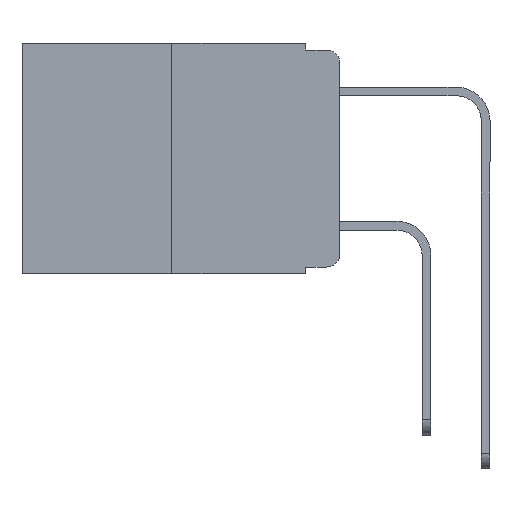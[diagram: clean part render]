
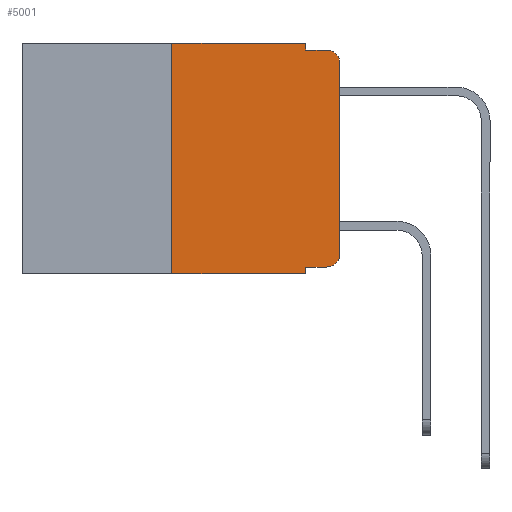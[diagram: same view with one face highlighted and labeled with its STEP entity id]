
A CAD part, left-side view. The second image highlights one B-rep face of the part: STEP entity #5001.
In plain terms, the highlighted planar face has unit normal (-1, 0, 0).
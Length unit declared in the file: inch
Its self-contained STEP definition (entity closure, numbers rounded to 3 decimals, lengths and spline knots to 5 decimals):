
#35 = ORIENTED_EDGE ( 'NONE', *, *, #887, .T. ) ;
#97 = VECTOR ( 'NONE', #2589, 39.37008 ) ;
#420 = DIRECTION ( 'NONE',  ( 0., 0., -1. ) ) ;
#448 = DIRECTION ( 'NONE',  ( 1., 0., 0. ) ) ;
#576 = VECTOR ( 'NONE', #7591, 39.37008 ) ;
#628 = CARTESIAN_POINT ( 'NONE',  ( 0., 0.051, 0. ) ) ;
#778 = LINE ( 'NONE', #7383, #7174 ) ;
#887 = EDGE_CURVE ( 'NONE', #8744, #9918, #8499, .T. ) ;
#1241 = CARTESIAN_POINT ( 'NONE',  ( 0., 0.051, -0.333 ) ) ;
#1350 = LINE ( 'NONE', #6227, #8189 ) ;
#1382 = CARTESIAN_POINT ( 'NONE',  ( 0., 0.02, -0.333 ) ) ;
#1446 = CARTESIAN_POINT ( 'NONE',  ( 0., 0., -0.313 ) ) ;
#1821 = DIRECTION ( 'NONE',  ( 0., -1., 0. ) ) ;
#2236 = PLANE ( 'NONE',  #8236 ) ;
#2323 = VERTEX_POINT ( 'NONE', #5712 ) ;
#2476 = CARTESIAN_POINT ( 'NONE',  ( 0., 0.25, -0.343 ) ) ;
#2589 = DIRECTION ( 'NONE',  ( 0., 0., -1. ) ) ;
#2742 = EDGE_CURVE ( 'NONE', #6399, #9145, #3777, .T. ) ;
#2753 = VERTEX_POINT ( 'NONE', #3191 ) ;
#2765 = CARTESIAN_POINT ( 'NONE',  ( 0., 0.02, -0.03 ) ) ;
#3017 = LINE ( 'NONE', #628, #576 ) ;
#3191 = CARTESIAN_POINT ( 'NONE',  ( 0., 0.25, 0. ) ) ;
#3298 = LINE ( 'NONE', #5934, #7515 ) ;
#3636 = DIRECTION ( 'NONE',  ( 0., 0., -1. ) ) ;
#3777 = LINE ( 'NONE', #4239, #6060 ) ;
#4095 = AXIS2_PLACEMENT_3D ( 'NONE', #2765, #8612, #3636 ) ;
#4237 = DIRECTION ( 'NONE',  ( -1., 0., 0. ) ) ;
#4239 = CARTESIAN_POINT ( 'NONE',  ( 0., 0.473, -0.343 ) ) ;
#4257 = FACE_OUTER_BOUND ( 'NONE', #5559, .T. ) ;
#4327 = VERTEX_POINT ( 'NONE', #1446 ) ;
#4471 = ORIENTED_EDGE ( 'NONE', *, *, #4555, .F. ) ;
#4555 = EDGE_CURVE ( 'NONE', #2323, #5750, #1350, .T. ) ;
#4623 = CARTESIAN_POINT ( 'NONE',  ( 0., 0.051, 0. ) ) ;
#4671 = EDGE_CURVE ( 'NONE', #2753, #8666, #778, .T. ) ;
#4885 = ORIENTED_EDGE ( 'NONE', *, *, #4671, .F. ) ;
#5001 = ADVANCED_FACE ( 'NONE', ( #4257 ), #2236, .F. ) ;
#5395 = ORIENTED_EDGE ( 'NONE', *, *, #9504, .F. ) ;
#5559 = EDGE_LOOP ( 'NONE', ( #5754, #6509, #4471, #5395, #4885, #10902, #8084, #10586, #35, #9125 ) ) ;
#5712 = CARTESIAN_POINT ( 'NONE',  ( 0., 0.051, -0.01 ) ) ;
#5750 = VERTEX_POINT ( 'NONE', #9078 ) ;
#5754 = ORIENTED_EDGE ( 'NONE', *, *, #9727, .T. ) ;
#5934 = CARTESIAN_POINT ( 'NONE',  ( 0., 0.25, 0. ) ) ;
#6060 = VECTOR ( 'NONE', #6420, 39.37008 ) ;
#6080 = DIRECTION ( 'NONE',  ( 0., -1., 0. ) ) ;
#6099 = CARTESIAN_POINT ( 'NONE',  ( 0., 0.473, 0. ) ) ;
#6188 = AXIS2_PLACEMENT_3D ( 'NONE', #9131, #4237, #9923 ) ;
#6193 = DIRECTION ( 'NONE',  ( 0., -1., 0. ) ) ;
#6227 = CARTESIAN_POINT ( 'NONE',  ( 0., 0.051, -0.01 ) ) ;
#6318 = DIRECTION ( 'NONE',  ( 0., 0., 1. ) ) ;
#6399 = VERTEX_POINT ( 'NONE', #2476 ) ;
#6420 = DIRECTION ( 'NONE',  ( 0., -1., 0. ) ) ;
#6509 = ORIENTED_EDGE ( 'NONE', *, *, #8564, .T. ) ;
#6766 = DIRECTION ( 'NONE',  ( 0., 0., 1. ) ) ;
#6854 = CARTESIAN_POINT ( 'NONE',  ( 0., 0.051, 0. ) ) ;
#6982 = VECTOR ( 'NONE', #6318, 39.37008 ) ;
#7131 = VECTOR ( 'NONE', #1821, 39.37008 ) ;
#7174 = VECTOR ( 'NONE', #6080, 39.37008 ) ;
#7383 = CARTESIAN_POINT ( 'NONE',  ( 0., 0.473, 0. ) ) ;
#7515 = VECTOR ( 'NONE', #6766, 39.37008 ) ;
#7591 = DIRECTION ( 'NONE',  ( 0., 0., -1. ) ) ;
#8084 = ORIENTED_EDGE ( 'NONE', *, *, #2742, .T. ) ;
#8189 = VECTOR ( 'NONE', #6193, 39.37008 ) ;
#8236 = AXIS2_PLACEMENT_3D ( 'NONE', #6099, #448, #420 ) ;
#8499 = LINE ( 'NONE', #8894, #7131 ) ;
#8564 = EDGE_CURVE ( 'NONE', #8829, #5750, #10442, .T. ) ;
#8612 = DIRECTION ( 'NONE',  ( -1., 0., 0. ) ) ;
#8666 = VERTEX_POINT ( 'NONE', #4623 ) ;
#8744 = VERTEX_POINT ( 'NONE', #1241 ) ;
#8829 = VERTEX_POINT ( 'NONE', #10611 ) ;
#8853 = EDGE_CURVE ( 'NONE', #6399, #2753, #3298, .T. ) ;
#8861 = EDGE_CURVE ( 'NONE', #9918, #4327, #9584, .T. ) ;
#8863 = EDGE_CURVE ( 'NONE', #8744, #9145, #3017, .T. ) ;
#8894 = CARTESIAN_POINT ( 'NONE',  ( 0., 0.051, -0.333 ) ) ;
#9068 = LINE ( 'NONE', #9452, #6982 ) ;
#9078 = CARTESIAN_POINT ( 'NONE',  ( 0., 0.02, -0.01 ) ) ;
#9125 = ORIENTED_EDGE ( 'NONE', *, *, #8861, .T. ) ;
#9131 = CARTESIAN_POINT ( 'NONE',  ( 0., 0.02, -0.313 ) ) ;
#9145 = VERTEX_POINT ( 'NONE', #10294 ) ;
#9192 = LINE ( 'NONE', #6854, #97 ) ;
#9452 = CARTESIAN_POINT ( 'NONE',  ( 0., 0., 0. ) ) ;
#9504 = EDGE_CURVE ( 'NONE', #8666, #2323, #9192, .T. ) ;
#9584 = CIRCLE ( 'NONE', #6188, 0.02 ) ;
#9727 = EDGE_CURVE ( 'NONE', #4327, #8829, #9068, .T. ) ;
#9918 = VERTEX_POINT ( 'NONE', #1382 ) ;
#9923 = DIRECTION ( 'NONE',  ( 0., 0., -1. ) ) ;
#10294 = CARTESIAN_POINT ( 'NONE',  ( 0., 0.051, -0.343 ) ) ;
#10442 = CIRCLE ( 'NONE', #4095, 0.02 ) ;
#10586 = ORIENTED_EDGE ( 'NONE', *, *, #8863, .F. ) ;
#10611 = CARTESIAN_POINT ( 'NONE',  ( 0., 0., -0.03 ) ) ;
#10902 = ORIENTED_EDGE ( 'NONE', *, *, #8853, .F. ) ;
